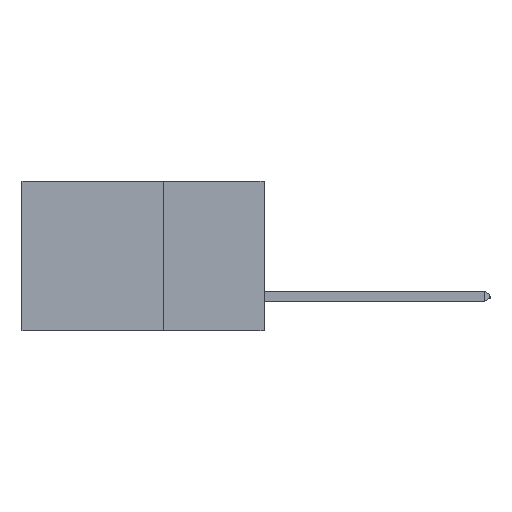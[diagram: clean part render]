
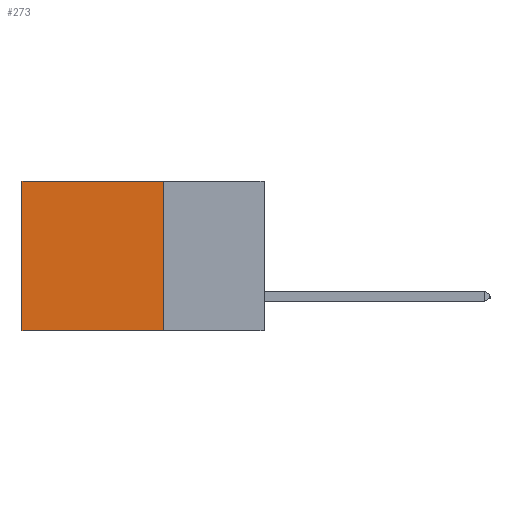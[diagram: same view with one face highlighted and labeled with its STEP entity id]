
A CAD part, left-side view. The second image highlights one B-rep face of the part: STEP entity #273.
In plain terms, the highlighted planar face has unit normal (-1, 0, 0).
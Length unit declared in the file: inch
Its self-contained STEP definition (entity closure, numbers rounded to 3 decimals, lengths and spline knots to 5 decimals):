
#273 = ADVANCED_FACE ( 'NONE', ( #15457 ), #6588, .F. ) ;
#1979 = CARTESIAN_POINT ( 'NONE',  ( 0.298, 0.25, 0. ) ) ;
#2427 = DIRECTION ( 'NONE',  ( 0., 0., -1. ) ) ;
#2686 = DIRECTION ( 'NONE',  ( 1., 0., 0. ) ) ;
#2854 = ORIENTED_EDGE ( 'NONE', *, *, #5259, .T. ) ;
#3683 = VECTOR ( 'NONE', #6906, 39.37008 ) ;
#5118 = CARTESIAN_POINT ( 'NONE',  ( 0.298, 0.25, -0.37 ) ) ;
#5259 = EDGE_CURVE ( 'NONE', #19157, #9575, #16907, .T. ) ;
#6529 = LINE ( 'NONE', #11806, #21411 ) ;
#6588 = PLANE ( 'NONE',  #7983 ) ;
#6906 = DIRECTION ( 'NONE',  ( 0., 0., -1. ) ) ;
#7618 = ORIENTED_EDGE ( 'NONE', *, *, #22856, .F. ) ;
#7983 = AXIS2_PLACEMENT_3D ( 'NONE', #1979, #2686, #2427 ) ;
#9051 = LINE ( 'NONE', #10899, #3683 ) ;
#9292 = VERTEX_POINT ( 'NONE', #12639 ) ;
#9537 = CARTESIAN_POINT ( 'NONE',  ( 0.298, 0.6, -0.37 ) ) ;
#9575 = VERTEX_POINT ( 'NONE', #25633 ) ;
#10886 = ORIENTED_EDGE ( 'NONE', *, *, #14847, .F. ) ;
#10899 = CARTESIAN_POINT ( 'NONE',  ( 0.298, 0.6, 0. ) ) ;
#11445 = VECTOR ( 'NONE', #21304, 39.37008 ) ;
#11526 = VECTOR ( 'NONE', #18713, 39.37008 ) ;
#11806 = CARTESIAN_POINT ( 'NONE',  ( 0.298, 0.25, 0. ) ) ;
#12497 = CARTESIAN_POINT ( 'NONE',  ( 0.298, 0.25, 0. ) ) ;
#12639 = CARTESIAN_POINT ( 'NONE',  ( 0.298, 0.25, -0.37 ) ) ;
#13846 = EDGE_LOOP ( 'NONE', ( #25328, #10886, #7618, #2854 ) ) ;
#14082 = EDGE_CURVE ( 'NONE', #9575, #14947, #9051, .T. ) ;
#14670 = CARTESIAN_POINT ( 'NONE',  ( 0.298, 0.25, 0. ) ) ;
#14847 = EDGE_CURVE ( 'NONE', #9292, #14947, #17458, .T. ) ;
#14947 = VERTEX_POINT ( 'NONE', #9537 ) ;
#15457 = FACE_OUTER_BOUND ( 'NONE', #13846, .T. ) ;
#15878 = DIRECTION ( 'NONE',  ( 0., 0., -1. ) ) ;
#16907 = LINE ( 'NONE', #14670, #11526 ) ;
#17458 = LINE ( 'NONE', #5118, #11445 ) ;
#18713 = DIRECTION ( 'NONE',  ( 0., 1., 0. ) ) ;
#19157 = VERTEX_POINT ( 'NONE', #12497 ) ;
#21304 = DIRECTION ( 'NONE',  ( 0., 1., 0. ) ) ;
#21411 = VECTOR ( 'NONE', #15878, 39.37008 ) ;
#22856 = EDGE_CURVE ( 'NONE', #19157, #9292, #6529, .T. ) ;
#25328 = ORIENTED_EDGE ( 'NONE', *, *, #14082, .T. ) ;
#25633 = CARTESIAN_POINT ( 'NONE',  ( 0.298, 0.6, 0. ) ) ;
